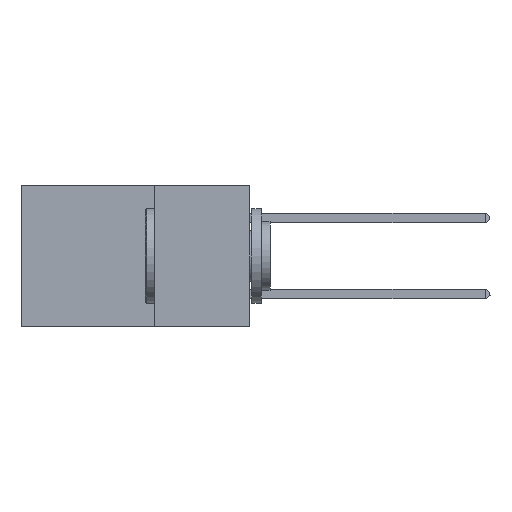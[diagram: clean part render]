
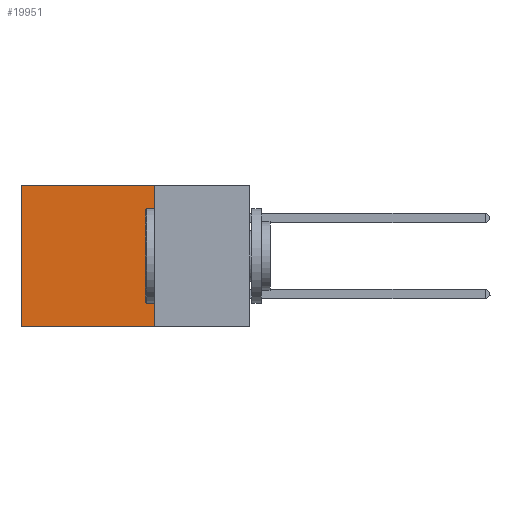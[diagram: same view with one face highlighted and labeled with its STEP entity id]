
A CAD part, left-side view. The second image highlights one B-rep face of the part: STEP entity #19951.
In plain terms, the highlighted planar face has unit normal (-1, 0, 0).
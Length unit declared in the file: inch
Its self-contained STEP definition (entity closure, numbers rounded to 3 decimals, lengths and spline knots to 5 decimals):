
#2929 = LINE ( 'NONE', #23521, #11596 ) ;
#2933 = DIRECTION ( 'NONE',  ( 1., 0., 0. ) ) ;
#6621 = LINE ( 'NONE', #21091, #40206 ) ;
#7282 = CARTESIAN_POINT ( 'NONE',  ( 0.2875, 0.25, -0.37 ) ) ;
#10484 = VECTOR ( 'NONE', #32723, 39.37008 ) ;
#10488 = EDGE_LOOP ( 'NONE', ( #12390, #31695, #24885, #21581 ) ) ;
#10536 = CARTESIAN_POINT ( 'NONE',  ( 0.2875, 0.6, 0. ) ) ;
#11596 = VECTOR ( 'NONE', #36628, 39.37008 ) ;
#11702 = VECTOR ( 'NONE', #19154, 39.37008 ) ;
#12390 = ORIENTED_EDGE ( 'NONE', *, *, #41270, .T. ) ;
#13468 = VERTEX_POINT ( 'NONE', #13978 ) ;
#13978 = CARTESIAN_POINT ( 'NONE',  ( 0.2875, 0.25, 0. ) ) ;
#14124 = DIRECTION ( 'NONE',  ( 0., 1., 0. ) ) ;
#15555 = VERTEX_POINT ( 'NONE', #10536 ) ;
#17694 = CARTESIAN_POINT ( 'NONE',  ( 0.2875, 0.6, -0.37 ) ) ;
#18629 = AXIS2_PLACEMENT_3D ( 'NONE', #19316, #2933, #35268 ) ;
#19154 = DIRECTION ( 'NONE',  ( 0., 1., 0. ) ) ;
#19316 = CARTESIAN_POINT ( 'NONE',  ( 0.2875, 0.25, 0. ) ) ;
#19951 = ADVANCED_FACE ( 'NONE', ( #37844 ), #22741, .F. ) ;
#20286 = VERTEX_POINT ( 'NONE', #17694 ) ;
#21091 = CARTESIAN_POINT ( 'NONE',  ( 0.2875, 0.25, -0.37 ) ) ;
#21581 = ORIENTED_EDGE ( 'NONE', *, *, #32941, .T. ) ;
#22020 = EDGE_CURVE ( 'NONE', #39393, #20286, #6621, .T. ) ;
#22173 = CARTESIAN_POINT ( 'NONE',  ( 0.2875, 0.25, 0. ) ) ;
#22741 = PLANE ( 'NONE',  #18629 ) ;
#23521 = CARTESIAN_POINT ( 'NONE',  ( 0.2875, 0.6, 0. ) ) ;
#24885 = ORIENTED_EDGE ( 'NONE', *, *, #41831, .F. ) ;
#29331 = LINE ( 'NONE', #35596, #10484 ) ;
#31695 = ORIENTED_EDGE ( 'NONE', *, *, #22020, .F. ) ;
#32723 = DIRECTION ( 'NONE',  ( 0., 0., -1. ) ) ;
#32941 = EDGE_CURVE ( 'NONE', #13468, #15555, #34616, .T. ) ;
#34616 = LINE ( 'NONE', #22173, #11702 ) ;
#35268 = DIRECTION ( 'NONE',  ( 0., 0., -1. ) ) ;
#35596 = CARTESIAN_POINT ( 'NONE',  ( 0.2875, 0.25, 0. ) ) ;
#36628 = DIRECTION ( 'NONE',  ( 0., 0., -1. ) ) ;
#37844 = FACE_OUTER_BOUND ( 'NONE', #10488, .T. ) ;
#39393 = VERTEX_POINT ( 'NONE', #7282 ) ;
#40206 = VECTOR ( 'NONE', #14124, 39.37008 ) ;
#41270 = EDGE_CURVE ( 'NONE', #15555, #20286, #2929, .T. ) ;
#41831 = EDGE_CURVE ( 'NONE', #13468, #39393, #29331, .T. ) ;
